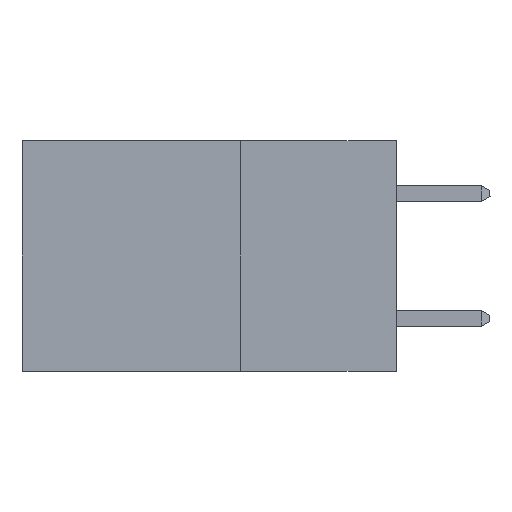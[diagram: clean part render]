
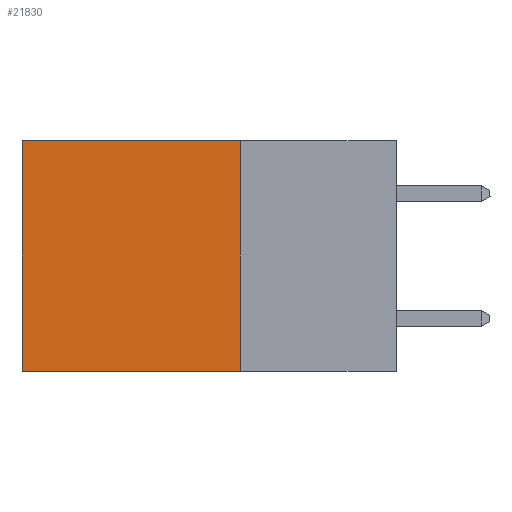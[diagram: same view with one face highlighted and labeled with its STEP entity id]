
A CAD part, left-side view. The second image highlights one B-rep face of the part: STEP entity #21830.
In plain terms, the highlighted planar face has unit normal (-1, 0, 0).
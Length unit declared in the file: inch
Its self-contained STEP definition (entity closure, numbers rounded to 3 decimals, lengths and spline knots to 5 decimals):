
#2282 = EDGE_CURVE ( 'NONE', #16324, #4705, #18138, .T. ) ;
#2451 = VECTOR ( 'NONE', #11002, 39.37008 ) ;
#4244 = CARTESIAN_POINT ( 'NONE',  ( 0.298, 0.25, 0. ) ) ;
#4705 = VERTEX_POINT ( 'NONE', #6991 ) ;
#4835 = DIRECTION ( 'NONE',  ( 1., 0., 0. ) ) ;
#5897 = CARTESIAN_POINT ( 'NONE',  ( 0.298, 0.25, 0. ) ) ;
#6615 = VERTEX_POINT ( 'NONE', #24324 ) ;
#6991 = CARTESIAN_POINT ( 'NONE',  ( 0.298, 0.6, -0.37 ) ) ;
#7040 = CARTESIAN_POINT ( 'NONE',  ( 0.298, 0.25, -0.37 ) ) ;
#8055 = EDGE_CURVE ( 'NONE', #18508, #16324, #23938, .T. ) ;
#8219 = ORIENTED_EDGE ( 'NONE', *, *, #14891, .T. ) ;
#8688 = CARTESIAN_POINT ( 'NONE',  ( 0.298, 0.25, 0. ) ) ;
#9430 = ORIENTED_EDGE ( 'NONE', *, *, #2282, .F. ) ;
#9838 = CARTESIAN_POINT ( 'NONE',  ( 0.298, 0.25, -0.37 ) ) ;
#10977 = DIRECTION ( 'NONE',  ( 0., 0., -1. ) ) ;
#11002 = DIRECTION ( 'NONE',  ( 0., 1., 0. ) ) ;
#11864 = VECTOR ( 'NONE', #17447, 39.37008 ) ;
#13920 = LINE ( 'NONE', #4244, #17325 ) ;
#14302 = DIRECTION ( 'NONE',  ( 0., 1., 0. ) ) ;
#14891 = EDGE_CURVE ( 'NONE', #18508, #6615, #13920, .T. ) ;
#15570 = FACE_OUTER_BOUND ( 'NONE', #18808, .T. ) ;
#16324 = VERTEX_POINT ( 'NONE', #9838 ) ;
#17325 = VECTOR ( 'NONE', #14302, 39.37008 ) ;
#17447 = DIRECTION ( 'NONE',  ( 0., 0., -1. ) ) ;
#18138 = LINE ( 'NONE', #7040, #2451 ) ;
#18419 = VECTOR ( 'NONE', #10977, 39.37008 ) ;
#18508 = VERTEX_POINT ( 'NONE', #5897 ) ;
#18808 = EDGE_LOOP ( 'NONE', ( #24592, #9430, #23963, #8219 ) ) ;
#19633 = EDGE_CURVE ( 'NONE', #6615, #4705, #19959, .T. ) ;
#19959 = LINE ( 'NONE', #20619, #18419 ) ;
#20490 = AXIS2_PLACEMENT_3D ( 'NONE', #8688, #4835, #22490 ) ;
#20504 = PLANE ( 'NONE',  #20490 ) ;
#20619 = CARTESIAN_POINT ( 'NONE',  ( 0.298, 0.6, 0. ) ) ;
#21830 = ADVANCED_FACE ( 'NONE', ( #15570 ), #20504, .F. ) ;
#22490 = DIRECTION ( 'NONE',  ( 0., 0., -1. ) ) ;
#23462 = CARTESIAN_POINT ( 'NONE',  ( 0.298, 0.25, 0. ) ) ;
#23938 = LINE ( 'NONE', #23462, #11864 ) ;
#23963 = ORIENTED_EDGE ( 'NONE', *, *, #8055, .F. ) ;
#24324 = CARTESIAN_POINT ( 'NONE',  ( 0.298, 0.6, 0. ) ) ;
#24592 = ORIENTED_EDGE ( 'NONE', *, *, #19633, .T. ) ;
